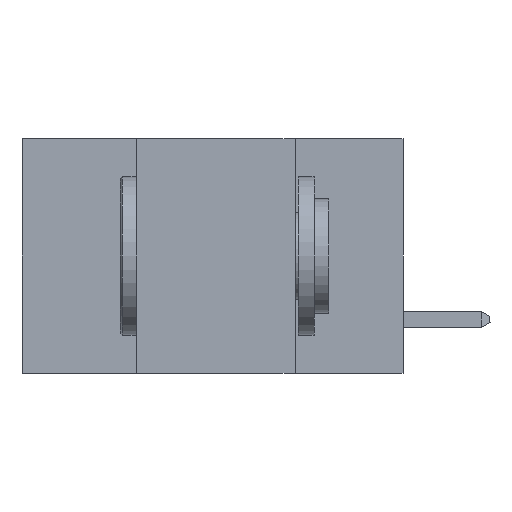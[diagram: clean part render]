
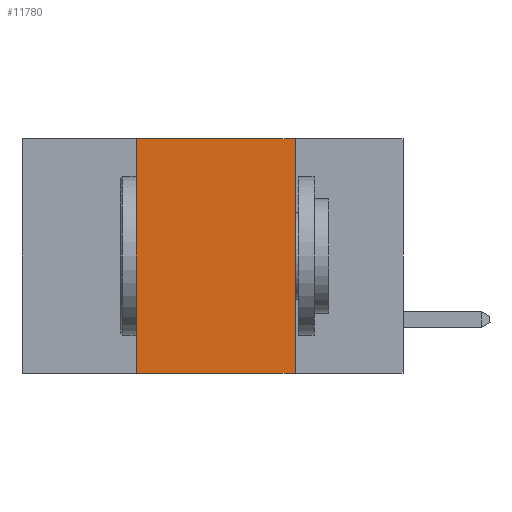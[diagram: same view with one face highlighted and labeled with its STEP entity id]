
A CAD part, left-side view. The second image highlights one B-rep face of the part: STEP entity #11780.
In plain terms, the highlighted planar face has unit normal (-1, 0, 0).
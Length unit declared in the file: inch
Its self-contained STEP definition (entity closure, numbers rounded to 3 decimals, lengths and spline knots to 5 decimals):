
#1393 = VECTOR ( 'NONE', #16922, 39.37008 ) ;
#1482 = VERTEX_POINT ( 'NONE', #2124 ) ;
#2124 = CARTESIAN_POINT ( 'NONE',  ( 0., 0.17, 0. ) ) ;
#2388 = PLANE ( 'NONE',  #7559 ) ;
#3204 = ORIENTED_EDGE ( 'NONE', *, *, #13047, .F. ) ;
#3538 = CARTESIAN_POINT ( 'NONE',  ( 0., 0.6, 0. ) ) ;
#3844 = DIRECTION ( 'NONE',  ( 0., 0., 1. ) ) ;
#4348 = ORIENTED_EDGE ( 'NONE', *, *, #13562, .T. ) ;
#4373 = VECTOR ( 'NONE', #3844, 39.37008 ) ;
#4548 = DIRECTION ( 'NONE',  ( 0., -1., 0. ) ) ;
#4821 = EDGE_LOOP ( 'NONE', ( #8256, #3204, #10373, #4348 ) ) ;
#4845 = EDGE_CURVE ( 'NONE', #1482, #12033, #15938, .T. ) ;
#5066 = VECTOR ( 'NONE', #7468, 39.37008 ) ;
#5874 = LINE ( 'NONE', #3538, #5066 ) ;
#7108 = EDGE_CURVE ( 'NONE', #16888, #15350, #9683, .T. ) ;
#7468 = DIRECTION ( 'NONE',  ( 0., -1., 0. ) ) ;
#7559 = AXIS2_PLACEMENT_3D ( 'NONE', #14043, #16892, #10318 ) ;
#7589 = CARTESIAN_POINT ( 'NONE',  ( 0., 0.42, 0. ) ) ;
#7650 = CARTESIAN_POINT ( 'NONE',  ( 0., 0.17, 0. ) ) ;
#8256 = ORIENTED_EDGE ( 'NONE', *, *, #4845, .F. ) ;
#9129 = VECTOR ( 'NONE', #4548, 39.37008 ) ;
#9199 = CARTESIAN_POINT ( 'NONE',  ( 0., 0.42, -0.37 ) ) ;
#9683 = LINE ( 'NONE', #7589, #4373 ) ;
#9809 = CARTESIAN_POINT ( 'NONE',  ( 0., 0.6, -0.37 ) ) ;
#10318 = DIRECTION ( 'NONE',  ( 0., 0., -1. ) ) ;
#10373 = ORIENTED_EDGE ( 'NONE', *, *, #7108, .F. ) ;
#11780 = ADVANCED_FACE ( 'NONE', ( #12820 ), #2388, .F. ) ;
#11944 = LINE ( 'NONE', #9809, #9129 ) ;
#12033 = VERTEX_POINT ( 'NONE', #16492 ) ;
#12430 = CARTESIAN_POINT ( 'NONE',  ( 0., 0.42, 0. ) ) ;
#12820 = FACE_OUTER_BOUND ( 'NONE', #4821, .T. ) ;
#13047 = EDGE_CURVE ( 'NONE', #15350, #1482, #5874, .T. ) ;
#13562 = EDGE_CURVE ( 'NONE', #16888, #12033, #11944, .T. ) ;
#14043 = CARTESIAN_POINT ( 'NONE',  ( 0., 0.6, 0. ) ) ;
#15350 = VERTEX_POINT ( 'NONE', #12430 ) ;
#15938 = LINE ( 'NONE', #7650, #1393 ) ;
#16492 = CARTESIAN_POINT ( 'NONE',  ( 0., 0.17, -0.37 ) ) ;
#16888 = VERTEX_POINT ( 'NONE', #9199 ) ;
#16892 = DIRECTION ( 'NONE',  ( 1., 0., 0. ) ) ;
#16922 = DIRECTION ( 'NONE',  ( 0., 0., -1. ) ) ;
